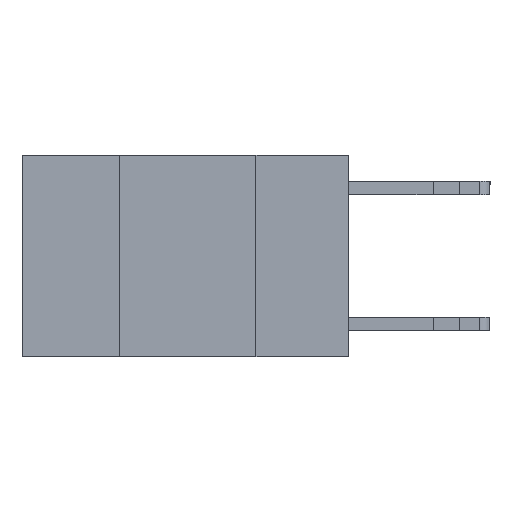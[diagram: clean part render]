
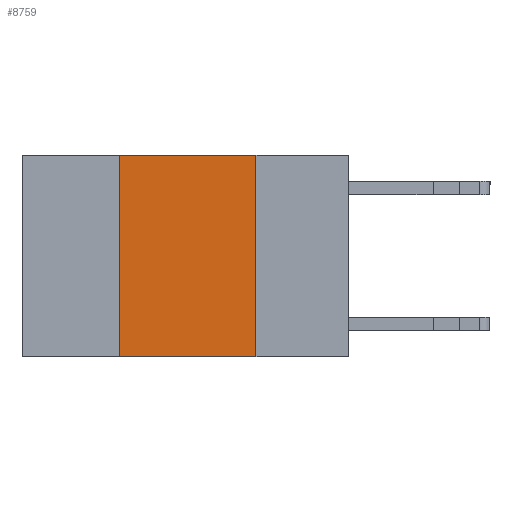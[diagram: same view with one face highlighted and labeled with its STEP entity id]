
A CAD part, left-side view. The second image highlights one B-rep face of the part: STEP entity #8759.
In plain terms, the highlighted planar face has unit normal (-1, 0, 0).
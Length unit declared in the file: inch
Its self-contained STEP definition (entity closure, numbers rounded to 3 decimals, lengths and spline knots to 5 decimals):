
#295 = VERTEX_POINT ( 'NONE', #4272 ) ;
#334 = PLANE ( 'NONE',  #13265 ) ;
#481 = EDGE_LOOP ( 'NONE', ( #2267, #713, #1233, #4817 ) ) ;
#713 = ORIENTED_EDGE ( 'NONE', *, *, #5950, .F. ) ;
#741 = DIRECTION ( 'NONE',  ( 0., 0., 1. ) ) ;
#1233 = ORIENTED_EDGE ( 'NONE', *, *, #10163, .F. ) ;
#1482 = FACE_OUTER_BOUND ( 'NONE', #481, .T. ) ;
#1652 = VERTEX_POINT ( 'NONE', #12954 ) ;
#1666 = CARTESIAN_POINT ( 'NONE',  ( 0., 0.17, 0. ) ) ;
#2267 = ORIENTED_EDGE ( 'NONE', *, *, #6567, .F. ) ;
#4272 = CARTESIAN_POINT ( 'NONE',  ( 0., 0.17, 0. ) ) ;
#4546 = LINE ( 'NONE', #12820, #7340 ) ;
#4621 = DIRECTION ( 'NONE',  ( 0., -1., 0. ) ) ;
#4817 = ORIENTED_EDGE ( 'NONE', *, *, #5482, .T. ) ;
#5091 = VERTEX_POINT ( 'NONE', #8793 ) ;
#5482 = EDGE_CURVE ( 'NONE', #5619, #1652, #4546, .T. ) ;
#5619 = VERTEX_POINT ( 'NONE', #8578 ) ;
#5950 = EDGE_CURVE ( 'NONE', #5091, #295, #11833, .T. ) ;
#6567 = EDGE_CURVE ( 'NONE', #295, #1652, #9678, .T. ) ;
#7071 = CARTESIAN_POINT ( 'NONE',  ( 0., 0.6, 0. ) ) ;
#7173 = VECTOR ( 'NONE', #741, 39.37008 ) ;
#7340 = VECTOR ( 'NONE', #4621, 39.37008 ) ;
#8320 = DIRECTION ( 'NONE',  ( 0., -1., 0. ) ) ;
#8578 = CARTESIAN_POINT ( 'NONE',  ( 0., 0.42, -0.37 ) ) ;
#8759 = ADVANCED_FACE ( 'NONE', ( #1482 ), #334, .F. ) ;
#8793 = CARTESIAN_POINT ( 'NONE',  ( 0., 0.42, 0. ) ) ;
#9190 = VECTOR ( 'NONE', #10967, 39.37008 ) ;
#9678 = LINE ( 'NONE', #1666, #9190 ) ;
#9806 = DIRECTION ( 'NONE',  ( 0., 0., -1. ) ) ;
#9831 = VECTOR ( 'NONE', #8320, 39.37008 ) ;
#10057 = LINE ( 'NONE', #14932, #7173 ) ;
#10163 = EDGE_CURVE ( 'NONE', #5619, #5091, #10057, .T. ) ;
#10939 = CARTESIAN_POINT ( 'NONE',  ( 0., 0.6, 0. ) ) ;
#10967 = DIRECTION ( 'NONE',  ( 0., 0., -1. ) ) ;
#11833 = LINE ( 'NONE', #7071, #9831 ) ;
#12820 = CARTESIAN_POINT ( 'NONE',  ( 0., 0.6, -0.37 ) ) ;
#12954 = CARTESIAN_POINT ( 'NONE',  ( 0., 0.17, -0.37 ) ) ;
#13244 = DIRECTION ( 'NONE',  ( 1., 0., 0. ) ) ;
#13265 = AXIS2_PLACEMENT_3D ( 'NONE', #10939, #13244, #9806 ) ;
#14932 = CARTESIAN_POINT ( 'NONE',  ( 0., 0.42, 0. ) ) ;
